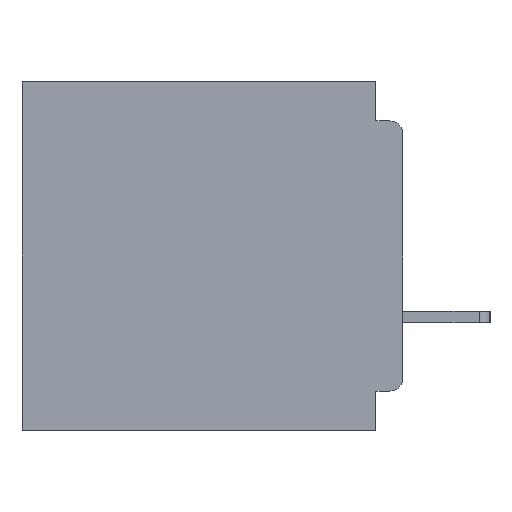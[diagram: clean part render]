
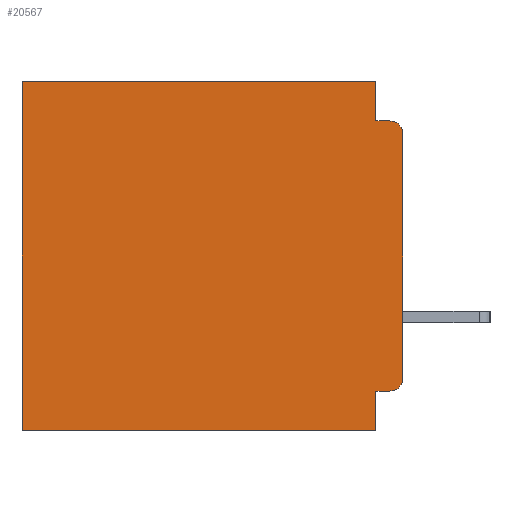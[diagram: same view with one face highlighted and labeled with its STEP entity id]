
A CAD part, left-side view. The second image highlights one B-rep face of the part: STEP entity #20567.
In plain terms, the highlighted planar face has unit normal (-1, 0, 0).
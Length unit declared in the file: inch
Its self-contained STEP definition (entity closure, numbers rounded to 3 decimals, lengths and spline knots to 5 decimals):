
#113 = DIRECTION ( 'NONE',  ( 0., 0., -1. ) ) ;
#683 = ORIENTED_EDGE ( 'NONE', *, *, #20503, .F. ) ;
#1026 = LINE ( 'NONE', #27563, #1984 ) ;
#1456 = VECTOR ( 'NONE', #33631, 39.37008 ) ;
#1653 = CARTESIAN_POINT ( 'NONE',  ( 0.3, 0.031, -0.4 ) ) ;
#1984 = VECTOR ( 'NONE', #9627, 39.37008 ) ;
#2108 = AXIS2_PLACEMENT_3D ( 'NONE', #35948, #18071, #113 ) ;
#2567 = VECTOR ( 'NONE', #28963, 39.37008 ) ;
#4004 = CARTESIAN_POINT ( 'NONE',  ( 0.3, 0., -0.4 ) ) ;
#4429 = LINE ( 'NONE', #28829, #2567 ) ;
#6451 = ORIENTED_EDGE ( 'NONE', *, *, #7996, .T. ) ;
#6534 = DIRECTION ( 'NONE',  ( 0., 1., 0. ) ) ;
#6854 = EDGE_CURVE ( 'NONE', #26235, #35578, #38369, .T. ) ;
#6985 = DIRECTION ( 'NONE',  ( 0., 0., -1. ) ) ;
#7060 = AXIS2_PLACEMENT_3D ( 'NONE', #31969, #14082, #34985 ) ;
#7112 = VERTEX_POINT ( 'NONE', #29007 ) ;
#7996 = EDGE_CURVE ( 'NONE', #13953, #29325, #28026, .T. ) ;
#8233 = VERTEX_POINT ( 'NONE', #9578 ) ;
#9578 = CARTESIAN_POINT ( 'NONE',  ( 0.3, 0.437, -0.4 ) ) ;
#9627 = DIRECTION ( 'NONE',  ( 0., 0., -1. ) ) ;
#10458 = EDGE_CURVE ( 'NONE', #37949, #16420, #20375, .T. ) ;
#11319 = LINE ( 'NONE', #27649, #1456 ) ;
#12396 = VECTOR ( 'NONE', #23549, 39.37008 ) ;
#12797 = CARTESIAN_POINT ( 'NONE',  ( 0.3, 0., -0.355 ) ) ;
#12974 = EDGE_CURVE ( 'NONE', #33629, #8233, #4429, .T. ) ;
#13953 = VERTEX_POINT ( 'NONE', #35742 ) ;
#14082 = DIRECTION ( 'NONE',  ( -1., 0., 0. ) ) ;
#14444 = CIRCLE ( 'NONE', #2108, 0.015 ) ;
#14526 = CARTESIAN_POINT ( 'NONE',  ( 0.3, 0., -0.045 ) ) ;
#14541 = VECTOR ( 'NONE', #24691, 39.37008 ) ;
#14547 = ORIENTED_EDGE ( 'NONE', *, *, #29971, .T. ) ;
#15531 = CARTESIAN_POINT ( 'NONE',  ( 0.3, 0.015, -0.355 ) ) ;
#15767 = EDGE_CURVE ( 'NONE', #29325, #8233, #34597, .T. ) ;
#16420 = VERTEX_POINT ( 'NONE', #24209 ) ;
#16824 = VECTOR ( 'NONE', #24000, 39.37008 ) ;
#17006 = LINE ( 'NONE', #1653, #31951 ) ;
#18071 = DIRECTION ( 'NONE',  ( -1., 0., 0. ) ) ;
#19382 = CARTESIAN_POINT ( 'NONE',  ( 0.3, 0.437, 0. ) ) ;
#19607 = DIRECTION ( 'NONE',  ( 0., 0., -1. ) ) ;
#20375 = LINE ( 'NONE', #14526, #12396 ) ;
#20503 = EDGE_CURVE ( 'NONE', #34173, #7112, #1026, .T. ) ;
#20567 = ADVANCED_FACE ( 'NONE', ( #29138 ), #33804, .F. ) ;
#20889 = ORIENTED_EDGE ( 'NONE', *, *, #12974, .F. ) ;
#21172 = EDGE_CURVE ( 'NONE', #13953, #37949, #11319, .T. ) ;
#22217 = CARTESIAN_POINT ( 'NONE',  ( 0.3, 0.031, -0.045 ) ) ;
#22971 = ORIENTED_EDGE ( 'NONE', *, *, #26467, .F. ) ;
#23549 = DIRECTION ( 'NONE',  ( 0., -1., 0. ) ) ;
#24000 = DIRECTION ( 'NONE',  ( 0., 0., -1. ) ) ;
#24166 = ORIENTED_EDGE ( 'NONE', *, *, #10458, .F. ) ;
#24209 = CARTESIAN_POINT ( 'NONE',  ( 0.3, 0.015, -0.045 ) ) ;
#24412 = CARTESIAN_POINT ( 'NONE',  ( 0.3, 0.031, -0.4 ) ) ;
#24466 = CARTESIAN_POINT ( 'NONE',  ( 0.3, 0., 0. ) ) ;
#24691 = DIRECTION ( 'NONE',  ( 0., 1., 0. ) ) ;
#24920 = DIRECTION ( 'NONE',  ( 1., 0., 0. ) ) ;
#26163 = EDGE_LOOP ( 'NONE', ( #683, #14547, #24166, #27168, #6451, #27287, #20889, #22971, #28201, #33458 ) ) ;
#26235 = VERTEX_POINT ( 'NONE', #15531 ) ;
#26467 = EDGE_CURVE ( 'NONE', #35578, #33629, #17006, .T. ) ;
#27168 = ORIENTED_EDGE ( 'NONE', *, *, #21172, .F. ) ;
#27287 = ORIENTED_EDGE ( 'NONE', *, *, #15767, .T. ) ;
#27563 = CARTESIAN_POINT ( 'NONE',  ( 0.3, 0., -0.4 ) ) ;
#27649 = CARTESIAN_POINT ( 'NONE',  ( 0.3, 0.031, 0. ) ) ;
#28026 = LINE ( 'NONE', #24466, #35953 ) ;
#28201 = ORIENTED_EDGE ( 'NONE', *, *, #6854, .F. ) ;
#28829 = CARTESIAN_POINT ( 'NONE',  ( 0.3, 0., -0.4 ) ) ;
#28963 = DIRECTION ( 'NONE',  ( 0., 1., 0. ) ) ;
#29007 = CARTESIAN_POINT ( 'NONE',  ( 0.3, 0., -0.34 ) ) ;
#29138 = FACE_OUTER_BOUND ( 'NONE', #26163, .T. ) ;
#29187 = CARTESIAN_POINT ( 'NONE',  ( 0.3, 0.031, -0.355 ) ) ;
#29325 = VERTEX_POINT ( 'NONE', #19382 ) ;
#29971 = EDGE_CURVE ( 'NONE', #34173, #16420, #35873, .T. ) ;
#31123 = EDGE_CURVE ( 'NONE', #26235, #7112, #14444, .T. ) ;
#31951 = VECTOR ( 'NONE', #19607, 39.37008 ) ;
#31969 = CARTESIAN_POINT ( 'NONE',  ( 0.3, 0.015, -0.06 ) ) ;
#32587 = AXIS2_PLACEMENT_3D ( 'NONE', #4004, #24920, #6985 ) ;
#32869 = CARTESIAN_POINT ( 'NONE',  ( 0.3, 0.437, -0.4 ) ) ;
#33458 = ORIENTED_EDGE ( 'NONE', *, *, #31123, .T. ) ;
#33629 = VERTEX_POINT ( 'NONE', #24412 ) ;
#33631 = DIRECTION ( 'NONE',  ( 0., 0., -1. ) ) ;
#33691 = CARTESIAN_POINT ( 'NONE',  ( 0.3, 0., -0.06 ) ) ;
#33804 = PLANE ( 'NONE',  #32587 ) ;
#34173 = VERTEX_POINT ( 'NONE', #33691 ) ;
#34597 = LINE ( 'NONE', #32869, #16824 ) ;
#34985 = DIRECTION ( 'NONE',  ( 0., 0., -1. ) ) ;
#35578 = VERTEX_POINT ( 'NONE', #29187 ) ;
#35742 = CARTESIAN_POINT ( 'NONE',  ( 0.3, 0.031, 0. ) ) ;
#35873 = CIRCLE ( 'NONE', #7060, 0.015 ) ;
#35948 = CARTESIAN_POINT ( 'NONE',  ( 0.3, 0.015, -0.34 ) ) ;
#35953 = VECTOR ( 'NONE', #6534, 39.37008 ) ;
#37949 = VERTEX_POINT ( 'NONE', #22217 ) ;
#38369 = LINE ( 'NONE', #12797, #14541 ) ;
